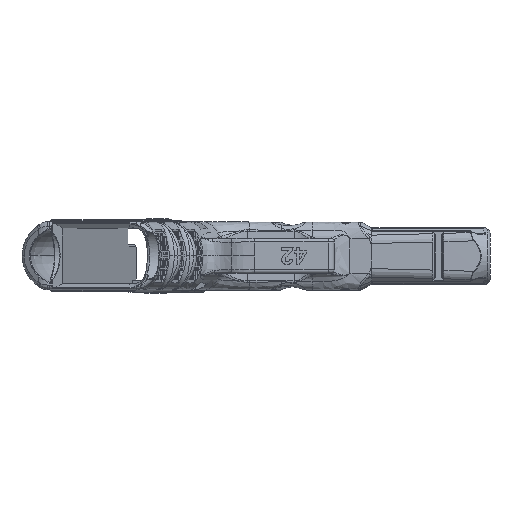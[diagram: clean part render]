
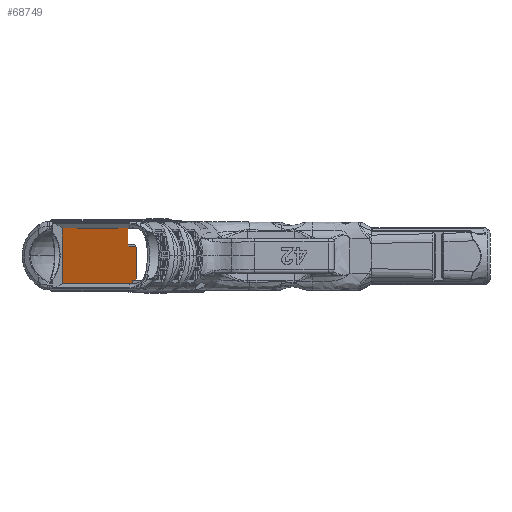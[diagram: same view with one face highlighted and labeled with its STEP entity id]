
A CAD part, top view. The second image highlights one B-rep face of the part: STEP entity #68749.
In plain terms, the highlighted planar face has unit normal (0.951, 0, 0.309).
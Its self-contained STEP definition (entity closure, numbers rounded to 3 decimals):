
#1262=ELLIPSE('',#72946,0.536,0.51);
#10901=FACE_OUTER_BOUND('',#14703,.T.);
#14703=EDGE_LOOP('',(#60377,#60378,#60379,#60380,#60381,#60382,#60383,#60384,
#60385,#60386,#60387));
#17447=LINE('',#130822,#22417);
#18584=LINE('',#191119,#23554);
#19579=LINE('',#204700,#24549);
#19582=LINE('',#204705,#24552);
#19587=LINE('',#204730,#24557);
#19588=LINE('',#204733,#24558);
#19589=LINE('',#204735,#24559);
#19590=LINE('',#204739,#24560);
#19591=LINE('',#204741,#24561);
#19592=LINE('',#204742,#24562);
#22417=VECTOR('',#79069,10.);
#23554=VECTOR('',#83148,10.);
#24549=VECTOR('',#84949,10.);
#24552=VECTOR('',#84956,10.);
#24557=VECTOR('',#84971,1000.);
#24558=VECTOR('',#84974,10.);
#24559=VECTOR('',#84975,10.);
#24560=VECTOR('',#84978,10.);
#24561=VECTOR('',#84979,10.);
#24562=VECTOR('',#84980,1000.);
#28147=VERTEX_POINT('',#130689);
#28163=VERTEX_POINT('',#130803);
#30221=VERTEX_POINT('',#191116);
#30222=VERTEX_POINT('',#191118);
#31327=VERTEX_POINT('',#204694);
#31329=VERTEX_POINT('',#204698);
#31337=VERTEX_POINT('',#204732);
#31338=VERTEX_POINT('',#204734);
#31339=VERTEX_POINT('',#204736);
#31340=VERTEX_POINT('',#204738);
#31341=VERTEX_POINT('',#204740);
#36393=EDGE_CURVE('',#28147,#28163,#17447,.T.);
#39575=EDGE_CURVE('',#30221,#30222,#18584,.T.);
#41247=EDGE_CURVE('',#31327,#31329,#19579,.T.);
#41250=EDGE_CURVE('',#31329,#30222,#19582,.T.);
#41260=EDGE_CURVE('',#31327,#28147,#19587,.T.);
#41261=EDGE_CURVE('',#31337,#30221,#19588,.T.);
#41262=EDGE_CURVE('',#31338,#31337,#19589,.T.);
#41263=EDGE_CURVE('',#31339,#31338,#1262,.T.);
#41264=EDGE_CURVE('',#31340,#31339,#19590,.T.);
#41265=EDGE_CURVE('',#31341,#31340,#19591,.T.);
#41266=EDGE_CURVE('',#28163,#31341,#19592,.T.);
#60377=ORIENTED_EDGE('',*,*,#41260,.F.);
#60378=ORIENTED_EDGE('',*,*,#41247,.T.);
#60379=ORIENTED_EDGE('',*,*,#41250,.T.);
#60380=ORIENTED_EDGE('',*,*,#39575,.F.);
#60381=ORIENTED_EDGE('',*,*,#41261,.F.);
#60382=ORIENTED_EDGE('',*,*,#41262,.F.);
#60383=ORIENTED_EDGE('',*,*,#41263,.F.);
#60384=ORIENTED_EDGE('',*,*,#41264,.F.);
#60385=ORIENTED_EDGE('',*,*,#41265,.F.);
#60386=ORIENTED_EDGE('',*,*,#41266,.F.);
#60387=ORIENTED_EDGE('',*,*,#36393,.F.);
#65471=PLANE('',#72945);
#68749=ADVANCED_FACE('',(#10901),#65471,.F.);
#72945=AXIS2_PLACEMENT_3D('',#204731,#84972,#84973);
#72946=AXIS2_PLACEMENT_3D('',#204737,#84976,#84977);
#79069=DIRECTION('',(0.,1.,0.));
#83148=DIRECTION('',(0.,-1.,0.));
#84949=DIRECTION('',(0.,1.,0.));
#84956=DIRECTION('',(0.309,0.,-0.951));
#84971=DIRECTION('',(-0.309,0.,0.951));
#84972=DIRECTION('center_axis',(-0.951,0.,
-0.309));
#84973=DIRECTION('ref_axis',(0.,1.,0.));
#84974=DIRECTION('',(-0.309,0.,0.951));
#84975=DIRECTION('',(0.,-1.,0.));
#84976=DIRECTION('center_axis',(-0.951,0.,
-0.309));
#84977=DIRECTION('ref_axis',(0.309,0.,-0.951));
#84978=DIRECTION('',(0.309,0.,-0.951));
#84979=DIRECTION('',(0.,-1.,0.));
#84980=DIRECTION('',(0.309,0.,-0.951));
#130689=CARTESIAN_POINT('',(2.236,-11.75,98.));
#130803=CARTESIAN_POINT('',(2.236,11.75,98.));
#130822=CARTESIAN_POINT('',(2.236,-18.375,98.));
#191116=CARTESIAN_POINT('',(33.331,-9.542,2.3));
#191118=CARTESIAN_POINT('',(33.331,-10.25,2.3));
#191119=CARTESIAN_POINT('',(33.331,-5.876,2.3));
#204694=CARTESIAN_POINT('',(31.8,-11.75,7.012));
#204698=CARTESIAN_POINT('',(31.8,-10.25,7.012));
#204700=CARTESIAN_POINT('',(31.8,-11.75,7.012));
#204705=CARTESIAN_POINT('',(33.225,-10.25,2.625));
#204730=CARTESIAN_POINT('',(33.829,-11.75,0.765));
#204731=CARTESIAN_POINT('Origin',(33.829,-11.75,0.765));
#204732=CARTESIAN_POINT('',(33.382,-9.542,2.141));
#204733=CARTESIAN_POINT('',(28.825,-9.542,16.167));
#204734=CARTESIAN_POINT('',(33.382,3.75,2.141));
#204735=CARTESIAN_POINT('',(33.382,-5.651,2.141));
#204736=CARTESIAN_POINT('',(33.216,4.26,2.651));
#204737=CARTESIAN_POINT('Origin',(33.216,3.75,2.651));
#204738=CARTESIAN_POINT('',(29.972,4.26,12.638));
#204739=CARTESIAN_POINT('',(34.619,4.26,-1.664));
#204740=CARTESIAN_POINT('',(29.972,11.75,12.638));
#204741=CARTESIAN_POINT('',(29.972,2.982,12.638));
#204742=CARTESIAN_POINT('',(30.125,11.75,12.165));
